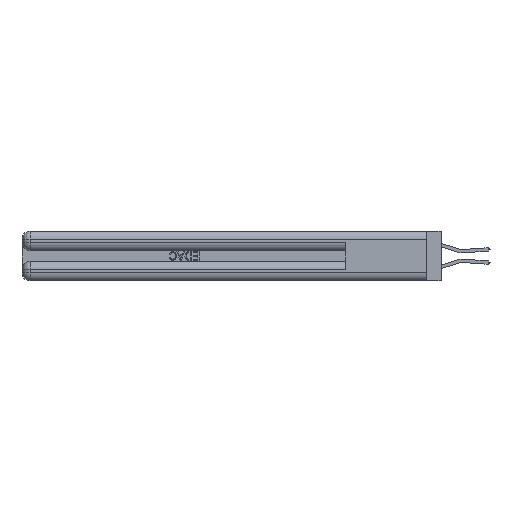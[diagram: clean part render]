
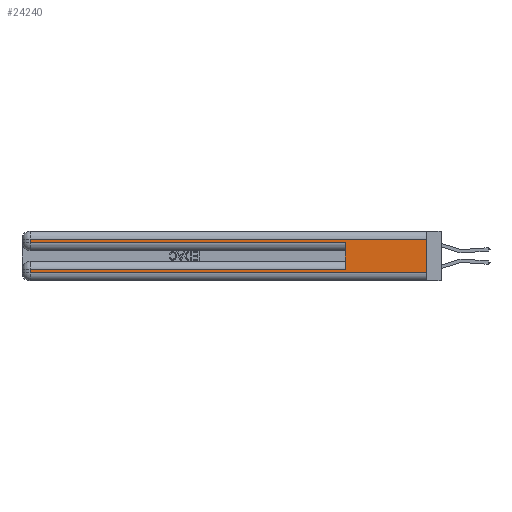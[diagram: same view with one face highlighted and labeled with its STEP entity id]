
A CAD part, left-side view. The second image highlights one B-rep face of the part: STEP entity #24240.
In plain terms, the highlighted planar face has unit normal (-1, 0, 0).
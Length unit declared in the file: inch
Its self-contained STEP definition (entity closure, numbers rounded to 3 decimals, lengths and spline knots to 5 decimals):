
#441 = CARTESIAN_POINT ( 'NONE',  ( 0., 0., 0.06 ) ) ;
#855 = ORIENTED_EDGE ( 'NONE', *, *, #11831, .T. ) ;
#1070 = VERTEX_POINT ( 'NONE', #31170 ) ;
#1102 = DIRECTION ( 'NONE',  ( 0., 1., 0. ) ) ;
#1429 = VERTEX_POINT ( 'NONE', #16024 ) ;
#3726 = CARTESIAN_POINT ( 'NONE',  ( 0., 2.94, 0.085 ) ) ;
#4944 = CARTESIAN_POINT ( 'NONE',  ( 0., 0.6, 0.145 ) ) ;
#5886 = CARTESIAN_POINT ( 'NONE',  ( 0., 0.6, 0.285 ) ) ;
#6207 = EDGE_CURVE ( 'NONE', #1429, #10857, #10240, .T. ) ;
#6266 = EDGE_CURVE ( 'NONE', #39529, #1070, #7487, .T. ) ;
#6860 = ORIENTED_EDGE ( 'NONE', *, *, #19559, .T. ) ;
#7022 = VECTOR ( 'NONE', #20335, 39.37008 ) ;
#7487 = LINE ( 'NONE', #13425, #13508 ) ;
#8669 = DIRECTION ( 'NONE',  ( 0., 0., -1. ) ) ;
#9633 = PLANE ( 'NONE',  #39814 ) ;
#10240 = LINE ( 'NONE', #4944, #14564 ) ;
#10354 = CARTESIAN_POINT ( 'NONE',  ( 0., 0., 0.31 ) ) ;
#10599 = CARTESIAN_POINT ( 'NONE',  ( 0., 2.94, 0.31 ) ) ;
#10857 = VERTEX_POINT ( 'NONE', #5886 ) ;
#11497 = EDGE_CURVE ( 'NONE', #32200, #21805, #35263, .T. ) ;
#11831 = EDGE_CURVE ( 'NONE', #1070, #10857, #16348, .T. ) ;
#12008 = VECTOR ( 'NONE', #43701, 39.37008 ) ;
#12056 = DIRECTION ( 'NONE',  ( 0., -1., 0. ) ) ;
#12534 = ORIENTED_EDGE ( 'NONE', *, *, #13387, .T. ) ;
#13245 = DIRECTION ( 'NONE',  ( 1., 0., 0. ) ) ;
#13387 = EDGE_CURVE ( 'NONE', #30239, #21805, #44881, .T. ) ;
#13425 = CARTESIAN_POINT ( 'NONE',  ( 0., 2.94, 0.37 ) ) ;
#13508 = VECTOR ( 'NONE', #44680, 39.37008 ) ;
#14564 = VECTOR ( 'NONE', #39375, 39.37008 ) ;
#14942 = CARTESIAN_POINT ( 'NONE',  ( 0., 0., 0.085 ) ) ;
#16024 = CARTESIAN_POINT ( 'NONE',  ( 0., 0.6, 0.085 ) ) ;
#16348 = LINE ( 'NONE', #27348, #7022 ) ;
#18459 = ORIENTED_EDGE ( 'NONE', *, *, #6207, .F. ) ;
#18556 = LINE ( 'NONE', #43861, #12008 ) ;
#19559 = EDGE_CURVE ( 'NONE', #1429, #27864, #30350, .T. ) ;
#19840 = CARTESIAN_POINT ( 'NONE',  ( 0., 0., 0.37 ) ) ;
#20144 = DIRECTION ( 'NONE',  ( 0., 0., -1. ) ) ;
#20335 = DIRECTION ( 'NONE',  ( 0., -1., 0. ) ) ;
#21805 = VERTEX_POINT ( 'NONE', #441 ) ;
#21947 = ORIENTED_EDGE ( 'NONE', *, *, #11497, .F. ) ;
#22740 = CARTESIAN_POINT ( 'NONE',  ( 0., 0., 0.06 ) ) ;
#22845 = VECTOR ( 'NONE', #8669, 39.37008 ) ;
#23762 = EDGE_CURVE ( 'NONE', #27864, #30239, #36731, .T. ) ;
#24240 = ADVANCED_FACE ( 'NONE', ( #37220 ), #9633, .F. ) ;
#24932 = ORIENTED_EDGE ( 'NONE', *, *, #29486, .T. ) ;
#25144 = DIRECTION ( 'NONE',  ( 0., 0., -1. ) ) ;
#26523 = VECTOR ( 'NONE', #12056, 39.37008 ) ;
#27348 = CARTESIAN_POINT ( 'NONE',  ( 0., 0., 0.285 ) ) ;
#27864 = VERTEX_POINT ( 'NONE', #3726 ) ;
#29486 = EDGE_CURVE ( 'NONE', #32200, #39529, #18556, .T. ) ;
#30239 = VERTEX_POINT ( 'NONE', #37610 ) ;
#30350 = LINE ( 'NONE', #14942, #33033 ) ;
#31170 = CARTESIAN_POINT ( 'NONE',  ( 0., 2.94, 0.285 ) ) ;
#32200 = VERTEX_POINT ( 'NONE', #10354 ) ;
#32369 = VECTOR ( 'NONE', #25144, 39.37008 ) ;
#33033 = VECTOR ( 'NONE', #1102, 39.37008 ) ;
#34544 = CARTESIAN_POINT ( 'NONE',  ( 0., 0., 0.37 ) ) ;
#35263 = LINE ( 'NONE', #34544, #22845 ) ;
#36731 = LINE ( 'NONE', #43026, #32369 ) ;
#37220 = FACE_OUTER_BOUND ( 'NONE', #41416, .T. ) ;
#37610 = CARTESIAN_POINT ( 'NONE',  ( 0., 2.94, 0.06 ) ) ;
#39375 = DIRECTION ( 'NONE',  ( 0., 0., 1. ) ) ;
#39529 = VERTEX_POINT ( 'NONE', #10599 ) ;
#39814 = AXIS2_PLACEMENT_3D ( 'NONE', #19840, #13245, #20144 ) ;
#40093 = ORIENTED_EDGE ( 'NONE', *, *, #23762, .T. ) ;
#41416 = EDGE_LOOP ( 'NONE', ( #21947, #24932, #42302, #855, #18459, #6860, #40093, #12534 ) ) ;
#42302 = ORIENTED_EDGE ( 'NONE', *, *, #6266, .T. ) ;
#43026 = CARTESIAN_POINT ( 'NONE',  ( 0., 2.94, 0.37 ) ) ;
#43701 = DIRECTION ( 'NONE',  ( 0., 1., 0. ) ) ;
#43861 = CARTESIAN_POINT ( 'NONE',  ( 0., 0., 0.31 ) ) ;
#44680 = DIRECTION ( 'NONE',  ( 0., 0., -1. ) ) ;
#44881 = LINE ( 'NONE', #22740, #26523 ) ;
